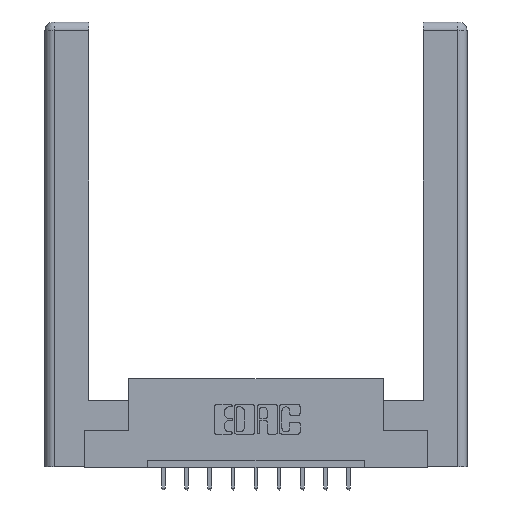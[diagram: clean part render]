
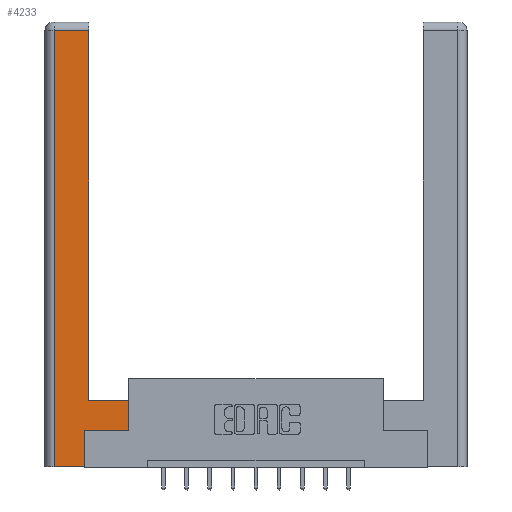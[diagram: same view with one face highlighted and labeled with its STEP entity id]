
A CAD part, top view. The second image highlights one B-rep face of the part: STEP entity #4233.
In plain terms, the highlighted planar face has unit normal (0, 0, 1).
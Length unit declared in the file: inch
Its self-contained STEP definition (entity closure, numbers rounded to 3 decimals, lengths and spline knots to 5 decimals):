
#459 = LINE ( 'NONE', #7561, #5920 ) ;
#722 = CARTESIAN_POINT ( 'NONE',  ( 0.295, 2.94, 0. ) ) ;
#834 = DIRECTION ( 'NONE',  ( -1., 0., 0. ) ) ;
#1035 = VERTEX_POINT ( 'NONE', #12120 ) ;
#1327 = CARTESIAN_POINT ( 'NONE',  ( 0.0615, 0., 0. ) ) ;
#1663 = DIRECTION ( 'NONE',  ( 0., 0., -1. ) ) ;
#2057 = VECTOR ( 'NONE', #12939, 39.37008 ) ;
#2076 = VERTEX_POINT ( 'NONE', #722 ) ;
#2140 = DIRECTION ( 'NONE',  ( 0., 1., 0. ) ) ;
#2426 = EDGE_LOOP ( 'NONE', ( #12198, #11528, #11734, #6990, #9562, #9063, #8606, #8627 ) ) ;
#2953 = VECTOR ( 'NONE', #9133, 39.37008 ) ;
#3172 = DIRECTION ( 'NONE',  ( 0., 1., 0. ) ) ;
#3434 = DIRECTION ( 'NONE',  ( 1., 0., 0. ) ) ;
#3578 = DIRECTION ( 'NONE',  ( 1., 0., 0. ) ) ;
#3595 = CARTESIAN_POINT ( 'NONE',  ( 0.565, 0.45, 0. ) ) ;
#3600 = LINE ( 'NONE', #5893, #2953 ) ;
#3821 = FACE_OUTER_BOUND ( 'NONE', #2426, .T. ) ;
#3918 = LINE ( 'NONE', #7368, #11321 ) ;
#4233 = ADVANCED_FACE ( 'NONE', ( #3821 ), #6950, .F. ) ;
#4288 = VERTEX_POINT ( 'NONE', #7862 ) ;
#4823 = LINE ( 'NONE', #12766, #12064 ) ;
#5084 = VERTEX_POINT ( 'NONE', #8820 ) ;
#5294 = EDGE_CURVE ( 'NONE', #2076, #4288, #7244, .T. ) ;
#5876 = EDGE_CURVE ( 'NONE', #10052, #5084, #3600, .T. ) ;
#5893 = CARTESIAN_POINT ( 'NONE',  ( 0.295, 0.45, 0. ) ) ;
#5920 = VECTOR ( 'NONE', #3172, 39.37008 ) ;
#6242 = LINE ( 'NONE', #7690, #12484 ) ;
#6851 = EDGE_CURVE ( 'NONE', #1035, #8891, #3918, .T. ) ;
#6950 = PLANE ( 'NONE',  #10464 ) ;
#6990 = ORIENTED_EDGE ( 'NONE', *, *, #8476, .T. ) ;
#7243 = VERTEX_POINT ( 'NONE', #11711 ) ;
#7244 = LINE ( 'NONE', #12529, #10211 ) ;
#7368 = CARTESIAN_POINT ( 'NONE',  ( 0.265, 0.245, 0. ) ) ;
#7561 = CARTESIAN_POINT ( 'NONE',  ( 0.565, 0.45, 0. ) ) ;
#7690 = CARTESIAN_POINT ( 'NONE',  ( 0.265, 0., 0. ) ) ;
#7862 = CARTESIAN_POINT ( 'NONE',  ( 0.0615, 2.94, 0. ) ) ;
#8035 = VERTEX_POINT ( 'NONE', #12149 ) ;
#8376 = EDGE_CURVE ( 'NONE', #8035, #10052, #459, .T. ) ;
#8476 = EDGE_CURVE ( 'NONE', #7243, #1035, #6242, .T. ) ;
#8606 = ORIENTED_EDGE ( 'NONE', *, *, #8376, .T. ) ;
#8627 = ORIENTED_EDGE ( 'NONE', *, *, #5876, .T. ) ;
#8820 = CARTESIAN_POINT ( 'NONE',  ( 0.295, 0.45, 0. ) ) ;
#8891 = VERTEX_POINT ( 'NONE', #9810 ) ;
#9063 = ORIENTED_EDGE ( 'NONE', *, *, #13131, .T. ) ;
#9133 = DIRECTION ( 'NONE',  ( -1., 0., 0. ) ) ;
#9562 = ORIENTED_EDGE ( 'NONE', *, *, #6851, .T. ) ;
#9601 = LINE ( 'NONE', #1327, #2057 ) ;
#9810 = CARTESIAN_POINT ( 'NONE',  ( 0.265, 0.245, 0. ) ) ;
#9905 = LINE ( 'NONE', #11878, #11717 ) ;
#10041 = CARTESIAN_POINT ( 'NONE',  ( 0., 0., 0. ) ) ;
#10052 = VERTEX_POINT ( 'NONE', #3595 ) ;
#10211 = VECTOR ( 'NONE', #834, 39.37008 ) ;
#10464 = AXIS2_PLACEMENT_3D ( 'NONE', #10041, #1663, #13121 ) ;
#11121 = EDGE_CURVE ( 'NONE', #4288, #7243, #9601, .T. ) ;
#11321 = VECTOR ( 'NONE', #2140, 39.37008 ) ;
#11528 = ORIENTED_EDGE ( 'NONE', *, *, #5294, .T. ) ;
#11711 = CARTESIAN_POINT ( 'NONE',  ( 0.0615, 0., 0. ) ) ;
#11717 = VECTOR ( 'NONE', #13446, 39.37008 ) ;
#11734 = ORIENTED_EDGE ( 'NONE', *, *, #11121, .T. ) ;
#11878 = CARTESIAN_POINT ( 'NONE',  ( 0.295, 3., 0. ) ) ;
#12064 = VECTOR ( 'NONE', #3434, 39.37008 ) ;
#12120 = CARTESIAN_POINT ( 'NONE',  ( 0.265, 0., 0. ) ) ;
#12149 = CARTESIAN_POINT ( 'NONE',  ( 0.565, 0.245, 0. ) ) ;
#12198 = ORIENTED_EDGE ( 'NONE', *, *, #12828, .T. ) ;
#12484 = VECTOR ( 'NONE', #3578, 39.37008 ) ;
#12529 = CARTESIAN_POINT ( 'NONE',  ( 0.0615, 2.94, 0. ) ) ;
#12766 = CARTESIAN_POINT ( 'NONE',  ( 0.565, 0.245, 0. ) ) ;
#12828 = EDGE_CURVE ( 'NONE', #5084, #2076, #9905, .T. ) ;
#12939 = DIRECTION ( 'NONE',  ( 0., -1., 0. ) ) ;
#13121 = DIRECTION ( 'NONE',  ( -1., 0., 0. ) ) ;
#13131 = EDGE_CURVE ( 'NONE', #8891, #8035, #4823, .T. ) ;
#13446 = DIRECTION ( 'NONE',  ( 0., 1., 0. ) ) ;
